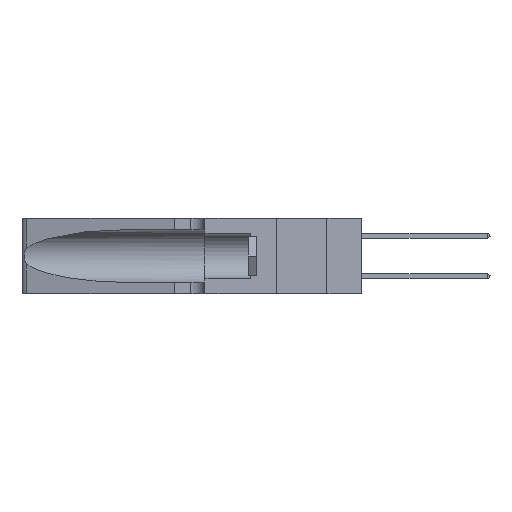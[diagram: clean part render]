
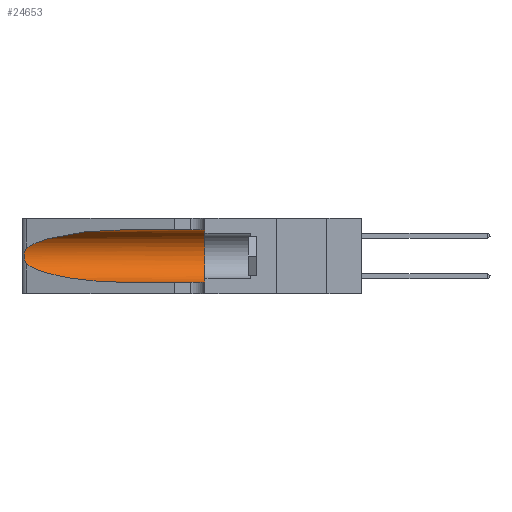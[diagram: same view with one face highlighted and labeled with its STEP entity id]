
A CAD part, left-side view. The second image highlights one B-rep face of the part: STEP entity #24653.
In plain terms, the highlighted cylindrical face has radius 3.308 mm (diameter 6.617 mm), a partial arc.
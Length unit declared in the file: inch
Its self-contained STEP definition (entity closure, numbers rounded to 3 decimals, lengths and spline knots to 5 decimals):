
#216 = DIRECTION ( 'NONE',  ( 0., -1., 0. ) ) ;
#303 = DIRECTION ( 'NONE',  ( 0., 1., 0. ) ) ;
#626 = ORIENTED_EDGE ( 'NONE', *, *, #20208, .T. ) ;
#718 = VERTEX_POINT ( 'NONE', #21235 ) ;
#941 = CARTESIAN_POINT ( 'NONE',  ( 0.26075, 1.23896, 0.178 ) ) ;
#996 = VERTEX_POINT ( 'NONE', #24369 ) ;
#2948 = CARTESIAN_POINT ( 'NONE',  ( 0.25856, 1.23593, 0.16098 ) ) ;
#4291 = CYLINDRICAL_SURFACE ( 'NONE', #9767, 0.13025 ) ;
#4511 = EDGE_CURVE ( 'NONE', #20792, #18608, #17076, .T. ) ;
#4902 = FACE_OUTER_BOUND ( 'NONE', #15272, .T. ) ;
#4928 = CARTESIAN_POINT ( 'NONE',  ( 0.25639, 1.23186, 0.15144 ) ) ;
#6834 = CARTESIAN_POINT ( 'NONE',  ( 0.25487, 1.22718, 0.22369 ) ) ;
#6923 = CARTESIAN_POINT ( 'NONE',  ( 0.25487, 1.22718, 0.14631 ) ) ;
#7242 = ORIENTED_EDGE ( 'NONE', *, *, #11423, .T. ) ;
#8427 = AXIS2_PLACEMENT_3D ( 'NONE', #12158, #303, #14144 ) ;
#8828 = CARTESIAN_POINT ( 'NONE',  ( 0.25639, 1.23184, 0.21858 ) ) ;
#8866 = VECTOR ( 'NONE', #17899, 39.37008 ) ;
#9625 = EDGE_CURVE ( 'NONE', #15201, #996, #15652, .T. ) ;
#9729 = CARTESIAN_POINT ( 'NONE',  ( 0.2373, 1.15595, 0.28018 ) ) ;
#9767 = AXIS2_PLACEMENT_3D ( 'NONE', #10080, #216, #14067 ) ;
#10080 = CARTESIAN_POINT ( 'NONE',  ( 0.1305, 1.61858, 0.185 ) ) ;
#10243 =( BOUNDED_CURVE ( )  B_SPLINE_CURVE ( 3, ( #19550, #25361, #9729, #23480 ),
 .UNSPECIFIED., .F., .T. ) 
 B_SPLINE_CURVE_WITH_KNOTS ( ( 4, 4 ),
 ( 1.5708, 2.84003 ),
 .UNSPECIFIED. ) 
 CURVE ( )  GEOMETRIC_REPRESENTATION_ITEM ( )  RATIONAL_B_SPLINE_CURVE ( ( 1., 0.87, 0.87, 1. ) ) 
 REPRESENTATION_ITEM ( '' )  );
#10800 = CARTESIAN_POINT ( 'NONE',  ( 0.25854, 1.2359, 0.20912 ) ) ;
#11030 = CARTESIAN_POINT ( 'NONE',  ( 0.1305, 0.72297, 0.05475 ) ) ;
#11423 = EDGE_CURVE ( 'NONE', #20792, #13997, #10243, .T. ) ;
#12057 = CARTESIAN_POINT ( 'NONE',  ( 0.1305, 1.61858, 0.05475 ) ) ;
#12158 = CARTESIAN_POINT ( 'NONE',  ( 0.1305, 0.35, 0.185 ) ) ;
#12559 = ORIENTED_EDGE ( 'NONE', *, *, #24676, .F. ) ;
#12788 = CARTESIAN_POINT ( 'NONE',  ( 0.26075, 1.23896, 0.19203 ) ) ;
#13679 = CARTESIAN_POINT ( 'NONE',  ( 0.25487, 1.22718, 0.22369 ) ) ;
#13997 = VERTEX_POINT ( 'NONE', #13679 ) ;
#14067 = DIRECTION ( 'NONE',  ( 0., 0., -1. ) ) ;
#14144 = DIRECTION ( 'NONE',  ( 0., 0., 1. ) ) ;
#14772 = CARTESIAN_POINT ( 'NONE',  ( 0.26017, 1.23833, 0.17102 ) ) ;
#15201 = VERTEX_POINT ( 'NONE', #20520 ) ;
#15272 = EDGE_LOOP ( 'NONE', ( #7242, #20038, #19538, #626, #12559, #24200 ) ) ;
#15652 =( BOUNDED_CURVE ( )  B_SPLINE_CURVE ( 3, ( #16883, #20838, #22808, #11030 ),
 .UNSPECIFIED., .F., .F. ) 
 B_SPLINE_CURVE_WITH_KNOTS ( ( 4, 4 ),
 ( 3.44316, 4.71239 ),
 .UNSPECIFIED. ) 
 CURVE ( )  GEOMETRIC_REPRESENTATION_ITEM ( )  RATIONAL_B_SPLINE_CURVE ( ( 1., 0.87, 0.87, 1. ) ) 
 REPRESENTATION_ITEM ( '' )  );
#16747 = CARTESIAN_POINT ( 'NONE',  ( 0.25789, 1.23486, 0.15765 ) ) ;
#16883 = CARTESIAN_POINT ( 'NONE',  ( 0.25487, 1.22718, 0.14631 ) ) ;
#17076 = LINE ( 'NONE', #22559, #20453 ) ;
#17899 = DIRECTION ( 'NONE',  ( 0., -1., 0. ) ) ;
#18608 = VERTEX_POINT ( 'NONE', #22609 ) ;
#18612 = DIRECTION ( 'NONE',  ( 0., -1., 0. ) ) ;
#18717 = CARTESIAN_POINT ( 'NONE',  ( 0.25555, 1.22993, 0.14849 ) ) ;
#19538 = ORIENTED_EDGE ( 'NONE', *, *, #9625, .T. ) ;
#19550 = CARTESIAN_POINT ( 'NONE',  ( 0.1305, 0.72297, 0.31525 ) ) ;
#19893 = CARTESIAN_POINT ( 'NONE',  ( 0.1305, 0.72297, 0.31525 ) ) ;
#20012 = CIRCLE ( 'NONE', #8427, 0.13025 ) ;
#20038 = ORIENTED_EDGE ( 'NONE', *, *, #21680, .T. ) ;
#20208 = EDGE_CURVE ( 'NONE', #996, #718, #23334, .T. ) ;
#20453 = VECTOR ( 'NONE', #18612, 39.37008 ) ;
#20520 = CARTESIAN_POINT ( 'NONE',  ( 0.25487, 1.22718, 0.14631 ) ) ;
#20792 = VERTEX_POINT ( 'NONE', #19893 ) ;
#20838 = CARTESIAN_POINT ( 'NONE',  ( 0.2373, 1.15595, 0.08982 ) ) ;
#21235 = CARTESIAN_POINT ( 'NONE',  ( 0.1305, 0.35, 0.05475 ) ) ;
#21680 = EDGE_CURVE ( 'NONE', #13997, #15201, #22528, .T. ) ;
#22528 = B_SPLINE_CURVE_WITH_KNOTS ( 'NONE', 3,
 ( #6834, #24473, #8828, #22587, #10800, #24557, #12788, #941, #14772, #2948, #16747, #4928, #18717, #6923 ),
 .UNSPECIFIED., .F., .F.,
 ( 4, 2, 2, 2, 2, 2, 4 ),
 ( 0., 0.00027, 0.00053, 0.00107, 0.0016, 0.00187, 0.00214 ),
 .UNSPECIFIED. ) ;
#22559 = CARTESIAN_POINT ( 'NONE',  ( 0.1305, 1.61858, 0.31525 ) ) ;
#22587 = CARTESIAN_POINT ( 'NONE',  ( 0.25787, 1.23484, 0.2124 ) ) ;
#22609 = CARTESIAN_POINT ( 'NONE',  ( 0.1305, 0.35, 0.31525 ) ) ;
#22808 = CARTESIAN_POINT ( 'NONE',  ( 0.18966, 0.96281, 0.05475 ) ) ;
#23334 = LINE ( 'NONE', #12057, #8866 ) ;
#23480 = CARTESIAN_POINT ( 'NONE',  ( 0.25487, 1.22718, 0.22369 ) ) ;
#24200 = ORIENTED_EDGE ( 'NONE', *, *, #4511, .F. ) ;
#24369 = CARTESIAN_POINT ( 'NONE',  ( 0.1305, 0.72297, 0.05475 ) ) ;
#24473 = CARTESIAN_POINT ( 'NONE',  ( 0.25555, 1.22994, 0.2215 ) ) ;
#24557 = CARTESIAN_POINT ( 'NONE',  ( 0.26018, 1.23835, 0.19895 ) ) ;
#24653 = ADVANCED_FACE ( 'NONE', ( #4902 ), #4291, .F. ) ;
#24676 = EDGE_CURVE ( 'NONE', #18608, #718, #20012, .T. ) ;
#25361 = CARTESIAN_POINT ( 'NONE',  ( 0.18966, 0.96281, 0.31525 ) ) ;
